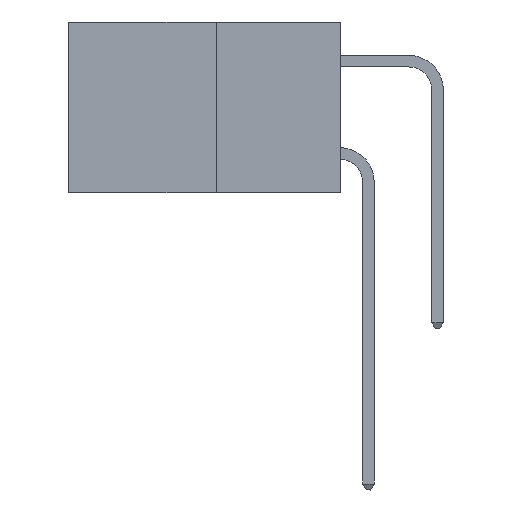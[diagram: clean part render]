
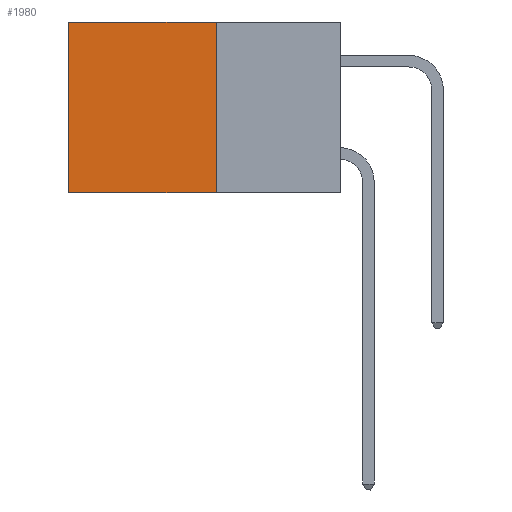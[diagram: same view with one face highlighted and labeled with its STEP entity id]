
A CAD part, left-side view. The second image highlights one B-rep face of the part: STEP entity #1980.
In plain terms, the highlighted planar face has unit normal (-1, 0, 0).
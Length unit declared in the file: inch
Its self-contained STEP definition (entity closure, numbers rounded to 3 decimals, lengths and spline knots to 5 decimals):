
#489 = DIRECTION ( 'NONE',  ( 0., 0., -1. ) ) ;
#1033 = DIRECTION ( 'NONE',  ( 0., 1., 0. ) ) ;
#1980 = ADVANCED_FACE ( 'NONE', ( #3066 ), #5175, .F. ) ;
#2150 = ORIENTED_EDGE ( 'NONE', *, *, #10553, .T. ) ;
#2169 = CARTESIAN_POINT ( 'NONE',  ( 0.277, 0.27, 0. ) ) ;
#2509 = ORIENTED_EDGE ( 'NONE', *, *, #3746, .F. ) ;
#2859 = CARTESIAN_POINT ( 'NONE',  ( 0.277, 0.59, 0. ) ) ;
#3066 = FACE_OUTER_BOUND ( 'NONE', #6346, .T. ) ;
#3114 = EDGE_CURVE ( 'NONE', #5873, #8154, #12069, .T. ) ;
#3195 = ORIENTED_EDGE ( 'NONE', *, *, #9314, .T. ) ;
#3427 = CARTESIAN_POINT ( 'NONE',  ( 0.277, 0.59, -0.37 ) ) ;
#3746 = EDGE_CURVE ( 'NONE', #8154, #9928, #13513, .T. ) ;
#3900 = CARTESIAN_POINT ( 'NONE',  ( 0.277, 0.27, -0.37 ) ) ;
#4341 = DIRECTION ( 'NONE',  ( 0., 1., 0. ) ) ;
#4351 = LINE ( 'NONE', #3427, #12203 ) ;
#4395 = LINE ( 'NONE', #2169, #12572 ) ;
#4632 = DIRECTION ( 'NONE',  ( 1., 0., 0. ) ) ;
#4638 = CARTESIAN_POINT ( 'NONE',  ( 0.277, 0.27, -0.37 ) ) ;
#4817 = DIRECTION ( 'NONE',  ( 0., 0., -1. ) ) ;
#5175 = PLANE ( 'NONE',  #5750 ) ;
#5750 = AXIS2_PLACEMENT_3D ( 'NONE', #3900, #4632, #4817 ) ;
#5873 = VERTEX_POINT ( 'NONE', #11292 ) ;
#6346 = EDGE_LOOP ( 'NONE', ( #2150, #2509, #11063, #3195 ) ) ;
#8154 = VERTEX_POINT ( 'NONE', #4638 ) ;
#9255 = VECTOR ( 'NONE', #489, 39.37008 ) ;
#9314 = EDGE_CURVE ( 'NONE', #5873, #12170, #4395, .T. ) ;
#9861 = CARTESIAN_POINT ( 'NONE',  ( 0.277, 0.27, -0.37 ) ) ;
#9928 = VERTEX_POINT ( 'NONE', #12698 ) ;
#10408 = VECTOR ( 'NONE', #4341, 39.37008 ) ;
#10553 = EDGE_CURVE ( 'NONE', #12170, #9928, #4351, .T. ) ;
#11063 = ORIENTED_EDGE ( 'NONE', *, *, #3114, .F. ) ;
#11075 = CARTESIAN_POINT ( 'NONE',  ( 0.277, 0.27, -0.37 ) ) ;
#11292 = CARTESIAN_POINT ( 'NONE',  ( 0.277, 0.27, 0. ) ) ;
#11973 = DIRECTION ( 'NONE',  ( 0., 0., -1. ) ) ;
#12069 = LINE ( 'NONE', #9861, #9255 ) ;
#12170 = VERTEX_POINT ( 'NONE', #2859 ) ;
#12203 = VECTOR ( 'NONE', #11973, 39.37008 ) ;
#12572 = VECTOR ( 'NONE', #1033, 39.37008 ) ;
#12698 = CARTESIAN_POINT ( 'NONE',  ( 0.277, 0.59, -0.37 ) ) ;
#13513 = LINE ( 'NONE', #11075, #10408 ) ;
